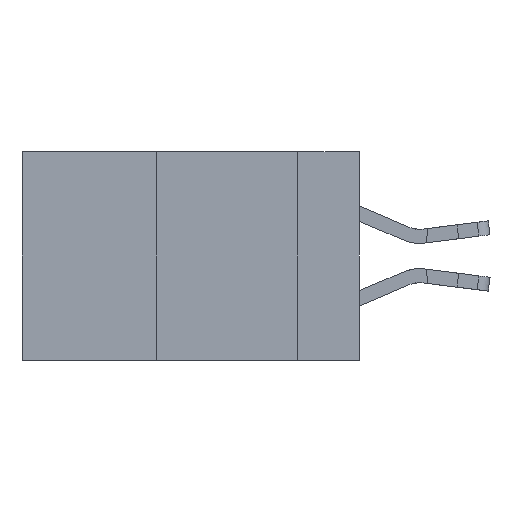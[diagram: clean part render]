
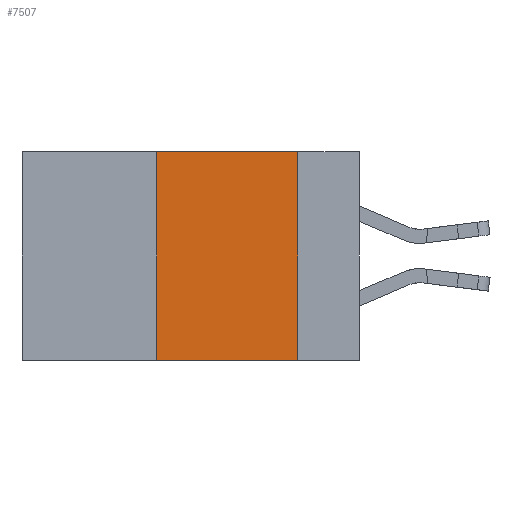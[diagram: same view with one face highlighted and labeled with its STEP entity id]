
A CAD part, left-side view. The second image highlights one B-rep face of the part: STEP entity #7507.
In plain terms, the highlighted planar face has unit normal (-1, 0, 0).
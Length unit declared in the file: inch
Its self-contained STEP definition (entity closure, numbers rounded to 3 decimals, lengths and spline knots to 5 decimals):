
#123 = VERTEX_POINT ( 'NONE', #4355 ) ;
#1631 = EDGE_CURVE ( 'NONE', #13878, #18796, #15871, .T. ) ;
#2098 = VECTOR ( 'NONE', #15109, 39.37008 ) ;
#2713 = EDGE_CURVE ( 'NONE', #13878, #123, #14460, .T. ) ;
#3499 = CARTESIAN_POINT ( 'NONE',  ( 0., 0.6, -0.37 ) ) ;
#4299 = DIRECTION ( 'NONE',  ( 0., 0., 1. ) ) ;
#4355 = CARTESIAN_POINT ( 'NONE',  ( 0., 0.11, -0.37 ) ) ;
#4450 = VECTOR ( 'NONE', #12742, 39.37008 ) ;
#4848 = ORIENTED_EDGE ( 'NONE', *, *, #1631, .F. ) ;
#5075 = ORIENTED_EDGE ( 'NONE', *, *, #12500, .F. ) ;
#7278 = CARTESIAN_POINT ( 'NONE',  ( 0., 0.36, 0. ) ) ;
#7507 = ADVANCED_FACE ( 'NONE', ( #18672 ), #12672, .F. ) ;
#7905 = VECTOR ( 'NONE', #4299, 39.37008 ) ;
#8169 = DIRECTION ( 'NONE',  ( 1., 0., 0. ) ) ;
#8409 = ORIENTED_EDGE ( 'NONE', *, *, #17199, .F. ) ;
#9539 = CARTESIAN_POINT ( 'NONE',  ( 0., 0.11, 0. ) ) ;
#9695 = CARTESIAN_POINT ( 'NONE',  ( 0., 0.11, 0. ) ) ;
#9779 = LINE ( 'NONE', #18095, #2098 ) ;
#9989 = VECTOR ( 'NONE', #12604, 39.37008 ) ;
#12452 = EDGE_LOOP ( 'NONE', ( #5075, #8409, #4848, #14301 ) ) ;
#12500 = EDGE_CURVE ( 'NONE', #17371, #123, #16913, .T. ) ;
#12604 = DIRECTION ( 'NONE',  ( 0., -1., 0. ) ) ;
#12672 = PLANE ( 'NONE',  #16472 ) ;
#12742 = DIRECTION ( 'NONE',  ( 0., 0., -1. ) ) ;
#12972 = CARTESIAN_POINT ( 'NONE',  ( 0., 0.36, 0. ) ) ;
#13878 = VERTEX_POINT ( 'NONE', #17697 ) ;
#14301 = ORIENTED_EDGE ( 'NONE', *, *, #2713, .T. ) ;
#14460 = LINE ( 'NONE', #3499, #9989 ) ;
#15109 = DIRECTION ( 'NONE',  ( 0., -1., 0. ) ) ;
#15637 = CARTESIAN_POINT ( 'NONE',  ( 0., 0.6, 0. ) ) ;
#15871 = LINE ( 'NONE', #7278, #7905 ) ;
#16472 = AXIS2_PLACEMENT_3D ( 'NONE', #15637, #8169, #18605 ) ;
#16913 = LINE ( 'NONE', #9695, #4450 ) ;
#17199 = EDGE_CURVE ( 'NONE', #18796, #17371, #9779, .T. ) ;
#17371 = VERTEX_POINT ( 'NONE', #9539 ) ;
#17697 = CARTESIAN_POINT ( 'NONE',  ( 0., 0.36, -0.37 ) ) ;
#18095 = CARTESIAN_POINT ( 'NONE',  ( 0., 0.6, 0. ) ) ;
#18605 = DIRECTION ( 'NONE',  ( 0., 0., -1. ) ) ;
#18672 = FACE_OUTER_BOUND ( 'NONE', #12452, .T. ) ;
#18796 = VERTEX_POINT ( 'NONE', #12972 ) ;
